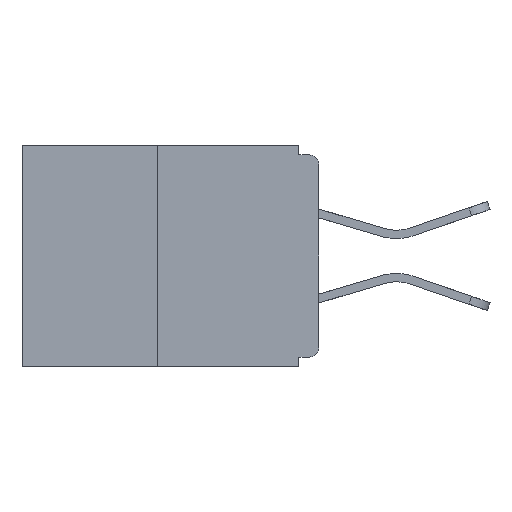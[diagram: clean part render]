
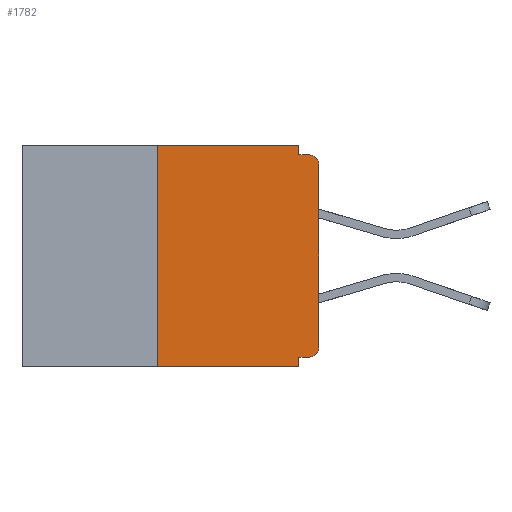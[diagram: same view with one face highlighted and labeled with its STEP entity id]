
A CAD part, left-side view. The second image highlights one B-rep face of the part: STEP entity #1782.
In plain terms, the highlighted planar face has unit normal (-1, 0, 0).
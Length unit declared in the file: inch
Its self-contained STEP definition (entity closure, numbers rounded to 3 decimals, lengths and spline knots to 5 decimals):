
#50 = CARTESIAN_POINT ( 'NONE',  ( 0., 0.46, -0.343 ) ) ;
#468 = CIRCLE ( 'NONE', #21856, 0.015 ) ;
#500 = EDGE_CURVE ( 'NONE', #17973, #8754, #27858, .T. ) ;
#1136 = ORIENTED_EDGE ( 'NONE', *, *, #6446, .T. ) ;
#1224 = LINE ( 'NONE', #26962, #16881 ) ;
#1409 = EDGE_LOOP ( 'NONE', ( #8445, #4474, #1136, #25564, #3627, #22640, #4304, #6176, #10332, #8822 ) ) ;
#1575 = CARTESIAN_POINT ( 'NONE',  ( 0., 0., 0. ) ) ;
#1734 = CARTESIAN_POINT ( 'NONE',  ( 0., 0.031, -0.015 ) ) ;
#1782 = ADVANCED_FACE ( 'NONE', ( #7613 ), #14317, .F. ) ;
#2357 = DIRECTION ( 'NONE',  ( 0., -1., 0. ) ) ;
#3198 = CARTESIAN_POINT ( 'NONE',  ( 0., 0.46, 0. ) ) ;
#3627 = ORIENTED_EDGE ( 'NONE', *, *, #16390, .F. ) ;
#4304 = ORIENTED_EDGE ( 'NONE', *, *, #21208, .T. ) ;
#4455 = VECTOR ( 'NONE', #2357, 39.37008 ) ;
#4474 = ORIENTED_EDGE ( 'NONE', *, *, #10779, .F. ) ;
#5131 = DIRECTION ( 'NONE',  ( 0., 0., -1. ) ) ;
#6176 = ORIENTED_EDGE ( 'NONE', *, *, #21157, .T. ) ;
#6446 = EDGE_CURVE ( 'NONE', #10145, #8754, #25347, .T. ) ;
#7095 = CARTESIAN_POINT ( 'NONE',  ( 0., 0.031, -0.343 ) ) ;
#7314 = CARTESIAN_POINT ( 'NONE',  ( 0., 0., -0.328 ) ) ;
#7613 = FACE_OUTER_BOUND ( 'NONE', #1409, .T. ) ;
#7699 = EDGE_CURVE ( 'NONE', #21544, #12528, #20055, .T. ) ;
#7847 = DIRECTION ( 'NONE',  ( 0., 0., 1. ) ) ;
#8246 = EDGE_CURVE ( 'NONE', #20248, #25042, #28039, .T. ) ;
#8342 = LINE ( 'NONE', #25719, #16687 ) ;
#8445 = ORIENTED_EDGE ( 'NONE', *, *, #7699, .F. ) ;
#8754 = VERTEX_POINT ( 'NONE', #11956 ) ;
#8822 = ORIENTED_EDGE ( 'NONE', *, *, #17142, .F. ) ;
#8910 = VECTOR ( 'NONE', #19524, 39.37008 ) ;
#8957 = CARTESIAN_POINT ( 'NONE',  ( 0., 0.015, -0.328 ) ) ;
#9168 = AXIS2_PLACEMENT_3D ( 'NONE', #3198, #18883, #5131 ) ;
#10055 = AXIS2_PLACEMENT_3D ( 'NONE', #18027, #22422, #26852 ) ;
#10145 = VERTEX_POINT ( 'NONE', #15321 ) ;
#10332 = ORIENTED_EDGE ( 'NONE', *, *, #25946, .F. ) ;
#10779 = EDGE_CURVE ( 'NONE', #10145, #21544, #26848, .T. ) ;
#11116 = CARTESIAN_POINT ( 'NONE',  ( 0., 0., -0.03 ) ) ;
#11821 = DIRECTION ( 'NONE',  ( 0., 1., 0. ) ) ;
#11956 = CARTESIAN_POINT ( 'NONE',  ( 0., 0.031, -0.343 ) ) ;
#12528 = VERTEX_POINT ( 'NONE', #26803 ) ;
#12902 = LINE ( 'NONE', #7314, #28205 ) ;
#13279 = VERTEX_POINT ( 'NONE', #11116 ) ;
#13733 = DIRECTION ( 'NONE',  ( 0., 0., -1. ) ) ;
#14267 = VERTEX_POINT ( 'NONE', #1734 ) ;
#14317 = PLANE ( 'NONE',  #9168 ) ;
#14847 = CARTESIAN_POINT ( 'NONE',  ( 0., 0.25, 0. ) ) ;
#15080 = DIRECTION ( 'NONE',  ( 0., 0., 1. ) ) ;
#15321 = CARTESIAN_POINT ( 'NONE',  ( 0., 0.25, -0.343 ) ) ;
#16390 = EDGE_CURVE ( 'NONE', #20248, #17973, #12902, .T. ) ;
#16687 = VECTOR ( 'NONE', #26100, 39.37008 ) ;
#16749 = DIRECTION ( 'NONE',  ( -1., 0., 0. ) ) ;
#16794 = LINE ( 'NONE', #1575, #25836 ) ;
#16881 = VECTOR ( 'NONE', #24861, 39.37008 ) ;
#17142 = EDGE_CURVE ( 'NONE', #12528, #14267, #8342, .T. ) ;
#17973 = VERTEX_POINT ( 'NONE', #21378 ) ;
#18027 = CARTESIAN_POINT ( 'NONE',  ( 0., 0.015, -0.313 ) ) ;
#18883 = DIRECTION ( 'NONE',  ( 1., 0., 0. ) ) ;
#19086 = CARTESIAN_POINT ( 'NONE',  ( 0., 0.015, -0.03 ) ) ;
#19324 = CARTESIAN_POINT ( 'NONE',  ( 0., 0.25, 0. ) ) ;
#19473 = CARTESIAN_POINT ( 'NONE',  ( 0., 0.015, -0.015 ) ) ;
#19524 = DIRECTION ( 'NONE',  ( 0., -1., 0. ) ) ;
#20055 = LINE ( 'NONE', #24298, #8910 ) ;
#20248 = VERTEX_POINT ( 'NONE', #8957 ) ;
#21157 = EDGE_CURVE ( 'NONE', #13279, #27456, #468, .T. ) ;
#21208 = EDGE_CURVE ( 'NONE', #25042, #13279, #16794, .T. ) ;
#21378 = CARTESIAN_POINT ( 'NONE',  ( 0., 0.031, -0.328 ) ) ;
#21544 = VERTEX_POINT ( 'NONE', #14847 ) ;
#21856 = AXIS2_PLACEMENT_3D ( 'NONE', #19086, #16749, #23590 ) ;
#22422 = DIRECTION ( 'NONE',  ( -1., 0., 0. ) ) ;
#22640 = ORIENTED_EDGE ( 'NONE', *, *, #8246, .T. ) ;
#22675 = VECTOR ( 'NONE', #13733, 39.37008 ) ;
#23590 = DIRECTION ( 'NONE',  ( 0., 0., -1. ) ) ;
#24298 = CARTESIAN_POINT ( 'NONE',  ( 0., 0.46, 0. ) ) ;
#24861 = DIRECTION ( 'NONE',  ( 0., -1., 0. ) ) ;
#25042 = VERTEX_POINT ( 'NONE', #27443 ) ;
#25347 = LINE ( 'NONE', #50, #4455 ) ;
#25564 = ORIENTED_EDGE ( 'NONE', *, *, #500, .F. ) ;
#25719 = CARTESIAN_POINT ( 'NONE',  ( 0., 0.031, 0. ) ) ;
#25836 = VECTOR ( 'NONE', #15080, 39.37008 ) ;
#25946 = EDGE_CURVE ( 'NONE', #14267, #27456, #1224, .T. ) ;
#26100 = DIRECTION ( 'NONE',  ( 0., 0., -1. ) ) ;
#26157 = VECTOR ( 'NONE', #7847, 39.37008 ) ;
#26803 = CARTESIAN_POINT ( 'NONE',  ( 0., 0.031, 0. ) ) ;
#26848 = LINE ( 'NONE', #19324, #26157 ) ;
#26852 = DIRECTION ( 'NONE',  ( 0., 0., -1. ) ) ;
#26962 = CARTESIAN_POINT ( 'NONE',  ( 0., 0., -0.015 ) ) ;
#27443 = CARTESIAN_POINT ( 'NONE',  ( 0., 0., -0.313 ) ) ;
#27456 = VERTEX_POINT ( 'NONE', #19473 ) ;
#27858 = LINE ( 'NONE', #7095, #22675 ) ;
#28039 = CIRCLE ( 'NONE', #10055, 0.015 ) ;
#28205 = VECTOR ( 'NONE', #11821, 39.37008 ) ;
